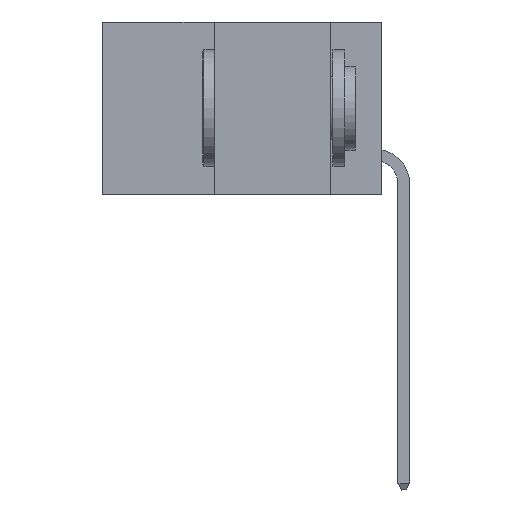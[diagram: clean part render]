
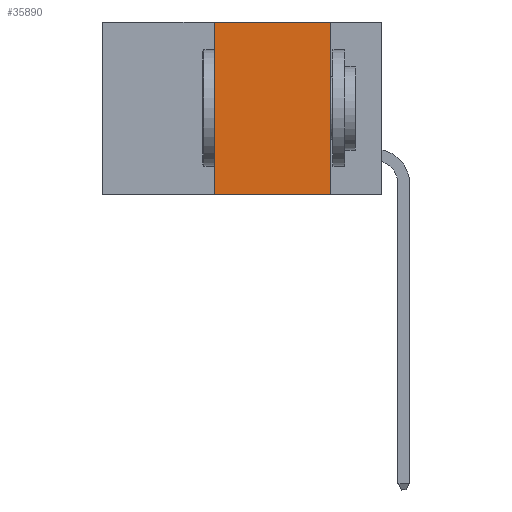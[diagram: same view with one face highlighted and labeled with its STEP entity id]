
A CAD part, left-side view. The second image highlights one B-rep face of the part: STEP entity #35890.
In plain terms, the highlighted planar face has unit normal (-1, 0, 0).
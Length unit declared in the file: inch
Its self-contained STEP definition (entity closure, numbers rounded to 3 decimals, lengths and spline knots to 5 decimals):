
#1321 = CARTESIAN_POINT ( 'NONE',  ( 0., 0.36, -0.37 ) ) ;
#2090 = ORIENTED_EDGE ( 'NONE', *, *, #14290, .T. ) ;
#5047 = ORIENTED_EDGE ( 'NONE', *, *, #24180, .F. ) ;
#6749 = VECTOR ( 'NONE', #22907, 39.37008 ) ;
#7173 = LINE ( 'NONE', #36943, #19059 ) ;
#8318 = CARTESIAN_POINT ( 'NONE',  ( 0., 0.36, 0. ) ) ;
#8665 = VERTEX_POINT ( 'NONE', #8318 ) ;
#9506 = DIRECTION ( 'NONE',  ( 0., 0., 1. ) ) ;
#9769 = VECTOR ( 'NONE', #23534, 39.37008 ) ;
#10148 = FACE_OUTER_BOUND ( 'NONE', #24789, .T. ) ;
#10405 = PLANE ( 'NONE',  #21717 ) ;
#12750 = CARTESIAN_POINT ( 'NONE',  ( 0., 0.11, 0. ) ) ;
#13512 = LINE ( 'NONE', #14030, #6749 ) ;
#14030 = CARTESIAN_POINT ( 'NONE',  ( 0., 0.6, 0. ) ) ;
#14290 = EDGE_CURVE ( 'NONE', #35002, #34454, #23069, .T. ) ;
#14525 = CARTESIAN_POINT ( 'NONE',  ( 0., 0.6, -0.37 ) ) ;
#16468 = DIRECTION ( 'NONE',  ( 1., 0., 0. ) ) ;
#16827 = LINE ( 'NONE', #12750, #28176 ) ;
#19059 = VECTOR ( 'NONE', #9506, 39.37008 ) ;
#21717 = AXIS2_PLACEMENT_3D ( 'NONE', #31575, #16468, #37695 ) ;
#21725 = DIRECTION ( 'NONE',  ( 0., 0., -1. ) ) ;
#22234 = VERTEX_POINT ( 'NONE', #33575 ) ;
#22907 = DIRECTION ( 'NONE',  ( 0., -1., 0. ) ) ;
#23069 = LINE ( 'NONE', #14525, #9769 ) ;
#23468 = ORIENTED_EDGE ( 'NONE', *, *, #32045, .F. ) ;
#23534 = DIRECTION ( 'NONE',  ( 0., -1., 0. ) ) ;
#24180 = EDGE_CURVE ( 'NONE', #22234, #34454, #16827, .T. ) ;
#24789 = EDGE_LOOP ( 'NONE', ( #5047, #23468, #37661, #2090 ) ) ;
#25280 = EDGE_CURVE ( 'NONE', #35002, #8665, #7173, .T. ) ;
#26014 = CARTESIAN_POINT ( 'NONE',  ( 0., 0.11, -0.37 ) ) ;
#28176 = VECTOR ( 'NONE', #21725, 39.37008 ) ;
#31575 = CARTESIAN_POINT ( 'NONE',  ( 0., 0.6, 0. ) ) ;
#32045 = EDGE_CURVE ( 'NONE', #8665, #22234, #13512, .T. ) ;
#33575 = CARTESIAN_POINT ( 'NONE',  ( 0., 0.11, 0. ) ) ;
#34454 = VERTEX_POINT ( 'NONE', #26014 ) ;
#35002 = VERTEX_POINT ( 'NONE', #1321 ) ;
#35890 = ADVANCED_FACE ( 'NONE', ( #10148 ), #10405, .F. ) ;
#36943 = CARTESIAN_POINT ( 'NONE',  ( 0., 0.36, 0. ) ) ;
#37661 = ORIENTED_EDGE ( 'NONE', *, *, #25280, .F. ) ;
#37695 = DIRECTION ( 'NONE',  ( 0., 0., -1. ) ) ;
